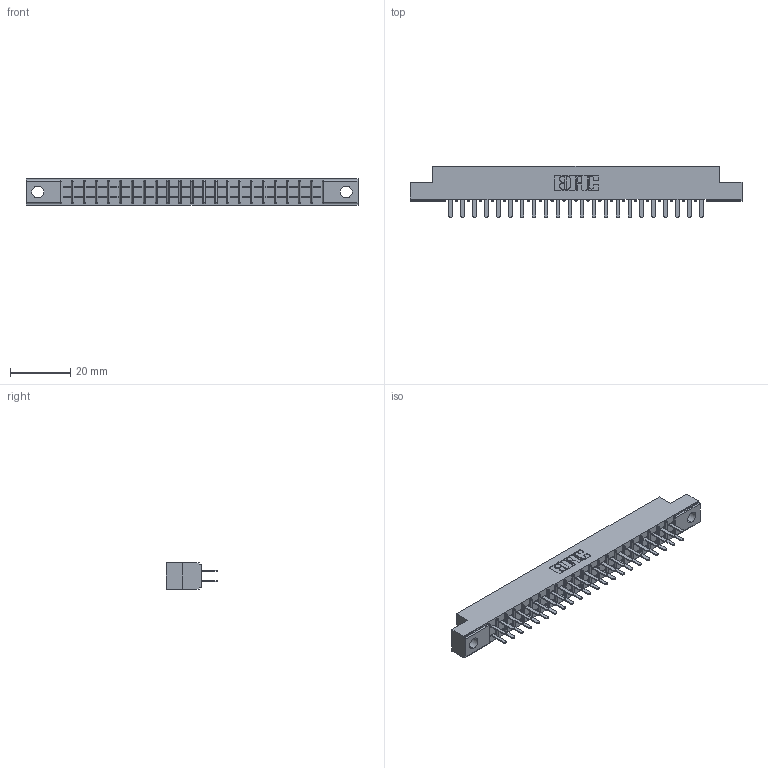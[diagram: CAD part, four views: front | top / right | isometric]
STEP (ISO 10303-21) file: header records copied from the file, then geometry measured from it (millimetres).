
FILE_DESCRIPTION (( 'STEP AP203' ), '1' );
FILE_NAME ('355-044-520-204.STEP', '2019-09-11T14:05:53', ( '' ), ( '' ), 'SwSTEP 2.0', 'SolidWorks 2016', '' );
FILE_SCHEMA (( 'CONFIG_CONTROL_DESIGN' ));
Length unit declared in the file: inch
Products named in the file (3): 305-290-001_520; 355-044-520-204; 305 Part_.156 Dia
Assembly tree (45 placements, depth 2):
  355-044-520-204
    305 Part_.156 Dia
    305-290-001_520  x44
Bounding box: 110.19 x 17.09 x 8.71 mm (x, y, z)
Volume: 6796.8 mm3; surface area: 12781.1 mm2
Topology: 45 solids, 45 shells, 2154 faces, 6138 edges, 3972 vertices
Faces by surface type: plane 1270, cylinder 796, sphere 88
Entity records: 26553 total; most frequent: CARTESIAN_POINT 4398, ORIENTED_EDGE 4360, DIRECTION 4262, EDGE_CURVE 2180, LINE 1750, VECTOR 1750, VERTEX_POINT 1392, AXIS2_PLACEMENT_3D 1256
